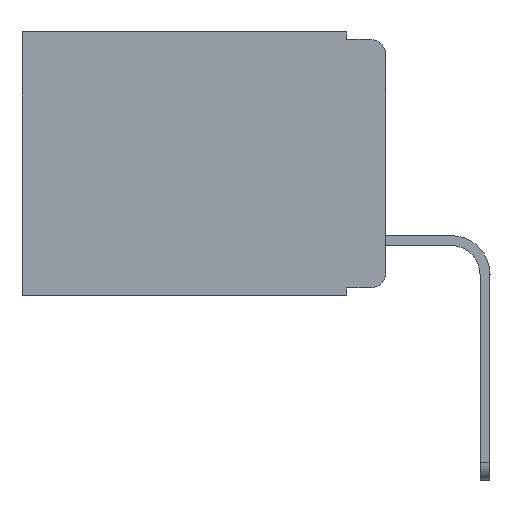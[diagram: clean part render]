
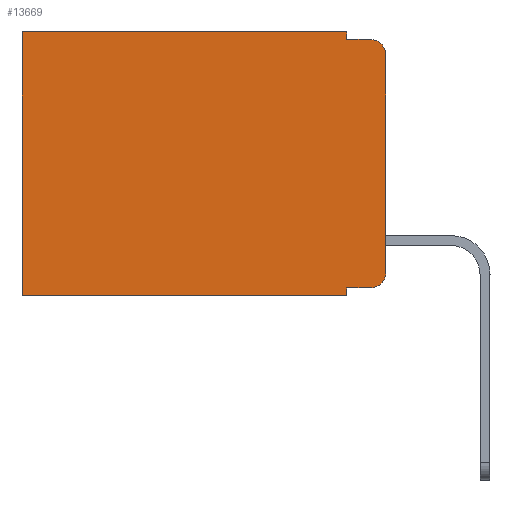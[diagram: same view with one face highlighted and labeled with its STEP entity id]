
A CAD part, left-side view. The second image highlights one B-rep face of the part: STEP entity #13669.
In plain terms, the highlighted planar face has unit normal (-1, 0, 0).
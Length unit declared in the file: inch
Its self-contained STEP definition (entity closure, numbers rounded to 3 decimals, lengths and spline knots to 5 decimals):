
#69 = VERTEX_POINT ( 'NONE', #1862 ) ;
#76 = VERTEX_POINT ( 'NONE', #3242 ) ;
#444 = DIRECTION ( 'NONE',  ( 0., -1., 0. ) ) ;
#596 = DIRECTION ( 'NONE',  ( 0., 0., -1. ) ) ;
#785 = FACE_OUTER_BOUND ( 'NONE', #15248, .T. ) ;
#1061 = ORIENTED_EDGE ( 'NONE', *, *, #7373, .F. ) ;
#1069 = ORIENTED_EDGE ( 'NONE', *, *, #15574, .T. ) ;
#1074 = LINE ( 'NONE', #1321, #3393 ) ;
#1100 = DIRECTION ( 'NONE',  ( 0., 0., -1. ) ) ;
#1161 = PLANE ( 'NONE',  #9991 ) ;
#1308 = CARTESIAN_POINT ( 'NONE',  ( 0.298, 0.051, -0.333 ) ) ;
#1321 = CARTESIAN_POINT ( 'NONE',  ( 0.298, 0.051, -0.01 ) ) ;
#1862 = CARTESIAN_POINT ( 'NONE',  ( 0.298, 0.051, -0.343 ) ) ;
#2124 = CARTESIAN_POINT ( 'NONE',  ( 0.298, 0.02, -0.313 ) ) ;
#2258 = LINE ( 'NONE', #4832, #4373 ) ;
#2263 = CARTESIAN_POINT ( 'NONE',  ( 0.298, 0.051, 0. ) ) ;
#2381 = EDGE_CURVE ( 'NONE', #17168, #69, #12424, .T. ) ;
#2947 = VERTEX_POINT ( 'NONE', #8576 ) ;
#3242 = CARTESIAN_POINT ( 'NONE',  ( 0.298, 0.473, 0. ) ) ;
#3393 = VECTOR ( 'NONE', #4098, 39.37008 ) ;
#3544 = CARTESIAN_POINT ( 'NONE',  ( 0.298, 0.051, 0. ) ) ;
#4098 = DIRECTION ( 'NONE',  ( 0., -1., 0. ) ) ;
#4373 = VECTOR ( 'NONE', #10076, 39.37008 ) ;
#4510 = EDGE_CURVE ( 'NONE', #2947, #15670, #1074, .T. ) ;
#4677 = CARTESIAN_POINT ( 'NONE',  ( 0.298, 0.473, -0.343 ) ) ;
#4770 = DIRECTION ( 'NONE',  ( -1., 0., 0. ) ) ;
#4832 = CARTESIAN_POINT ( 'NONE',  ( 0.298, 0., -0.343 ) ) ;
#4839 = CIRCLE ( 'NONE', #14883, 0.02 ) ;
#4874 = EDGE_CURVE ( 'NONE', #76, #7216, #12921, .T. ) ;
#5044 = CARTESIAN_POINT ( 'NONE',  ( 0.298, 0., -0.313 ) ) ;
#5286 = DIRECTION ( 'NONE',  ( 0., 0., -1. ) ) ;
#5386 = LINE ( 'NONE', #2263, #10680 ) ;
#5607 = ORIENTED_EDGE ( 'NONE', *, *, #12806, .F. ) ;
#5752 = CARTESIAN_POINT ( 'NONE',  ( 0.298, 0.051, -0.333 ) ) ;
#5998 = VERTEX_POINT ( 'NONE', #5044 ) ;
#6016 = VECTOR ( 'NONE', #444, 39.37008 ) ;
#6061 = LINE ( 'NONE', #9889, #13667 ) ;
#6289 = CARTESIAN_POINT ( 'NONE',  ( 0.298, 0., -0.03 ) ) ;
#6362 = VECTOR ( 'NONE', #11721, 39.37008 ) ;
#6492 = ORIENTED_EDGE ( 'NONE', *, *, #7538, .T. ) ;
#6586 = ORIENTED_EDGE ( 'NONE', *, *, #10908, .T. ) ;
#6608 = CARTESIAN_POINT ( 'NONE',  ( 0.298, 0.02, -0.03 ) ) ;
#7216 = VERTEX_POINT ( 'NONE', #4677 ) ;
#7373 = EDGE_CURVE ( 'NONE', #12860, #5998, #14975, .T. ) ;
#7538 = EDGE_CURVE ( 'NONE', #9035, #5998, #4839, .T. ) ;
#8025 = DIRECTION ( 'NONE',  ( 1., 0., 0. ) ) ;
#8576 = CARTESIAN_POINT ( 'NONE',  ( 0.298, 0.051, -0.01 ) ) ;
#8632 = CARTESIAN_POINT ( 'NONE',  ( 0.298, 0.02, -0.01 ) ) ;
#8777 = EDGE_CURVE ( 'NONE', #69, #7216, #2258, .T. ) ;
#9035 = VERTEX_POINT ( 'NONE', #14735 ) ;
#9066 = ORIENTED_EDGE ( 'NONE', *, *, #8777, .F. ) ;
#9161 = LINE ( 'NONE', #5752, #6016 ) ;
#9218 = CARTESIAN_POINT ( 'NONE',  ( 0.298, 0.473, 0. ) ) ;
#9889 = CARTESIAN_POINT ( 'NONE',  ( 0.298, 0., 0. ) ) ;
#9949 = DIRECTION ( 'NONE',  ( 0., 1., 0. ) ) ;
#9991 = AXIS2_PLACEMENT_3D ( 'NONE', #10734, #8025, #10646 ) ;
#10076 = DIRECTION ( 'NONE',  ( 0., 1., 0. ) ) ;
#10159 = VECTOR ( 'NONE', #596, 39.37008 ) ;
#10163 = ORIENTED_EDGE ( 'NONE', *, *, #2381, .F. ) ;
#10646 = DIRECTION ( 'NONE',  ( 0., 0., -1. ) ) ;
#10680 = VECTOR ( 'NONE', #11551, 39.37008 ) ;
#10734 = CARTESIAN_POINT ( 'NONE',  ( 0.298, 0., 0. ) ) ;
#10762 = VERTEX_POINT ( 'NONE', #3544 ) ;
#10908 = EDGE_CURVE ( 'NONE', #12860, #15670, #16099, .T. ) ;
#11551 = DIRECTION ( 'NONE',  ( 0., 0., -1. ) ) ;
#11721 = DIRECTION ( 'NONE',  ( 0., 0., -1. ) ) ;
#11995 = AXIS2_PLACEMENT_3D ( 'NONE', #6608, #17405, #5286 ) ;
#11997 = VECTOR ( 'NONE', #16341, 39.37008 ) ;
#12309 = ORIENTED_EDGE ( 'NONE', *, *, #4874, .T. ) ;
#12424 = LINE ( 'NONE', #12511, #11997 ) ;
#12511 = CARTESIAN_POINT ( 'NONE',  ( 0.298, 0.051, 0. ) ) ;
#12806 = EDGE_CURVE ( 'NONE', #10762, #2947, #5386, .T. ) ;
#12860 = VERTEX_POINT ( 'NONE', #6289 ) ;
#12921 = LINE ( 'NONE', #9218, #6362 ) ;
#13305 = EDGE_CURVE ( 'NONE', #10762, #76, #6061, .T. ) ;
#13384 = ORIENTED_EDGE ( 'NONE', *, *, #13305, .T. ) ;
#13667 = VECTOR ( 'NONE', #9949, 39.37008 ) ;
#13669 = ADVANCED_FACE ( 'NONE', ( #785 ), #1161, .F. ) ;
#13931 = CARTESIAN_POINT ( 'NONE',  ( 0.298, 0., 0. ) ) ;
#14735 = CARTESIAN_POINT ( 'NONE',  ( 0.298, 0.02, -0.333 ) ) ;
#14883 = AXIS2_PLACEMENT_3D ( 'NONE', #2124, #4770, #1100 ) ;
#14975 = LINE ( 'NONE', #13931, #10159 ) ;
#15229 = ORIENTED_EDGE ( 'NONE', *, *, #4510, .F. ) ;
#15248 = EDGE_LOOP ( 'NONE', ( #1061, #6586, #15229, #5607, #13384, #12309, #9066, #10163, #1069, #6492 ) ) ;
#15574 = EDGE_CURVE ( 'NONE', #17168, #9035, #9161, .T. ) ;
#15670 = VERTEX_POINT ( 'NONE', #8632 ) ;
#16099 = CIRCLE ( 'NONE', #11995, 0.02 ) ;
#16341 = DIRECTION ( 'NONE',  ( 0., 0., -1. ) ) ;
#17168 = VERTEX_POINT ( 'NONE', #1308 ) ;
#17405 = DIRECTION ( 'NONE',  ( -1., 0., 0. ) ) ;
